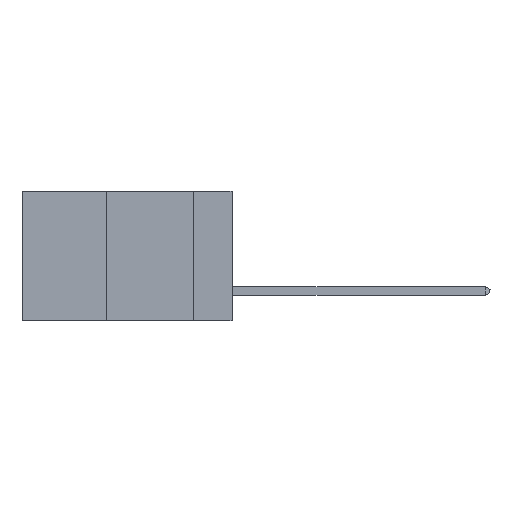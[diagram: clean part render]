
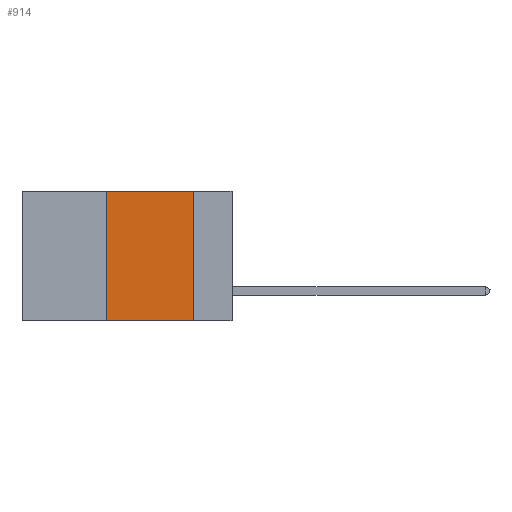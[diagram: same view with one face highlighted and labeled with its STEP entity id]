
A CAD part, left-side view. The second image highlights one B-rep face of the part: STEP entity #914.
In plain terms, the highlighted planar face has unit normal (-1, 0, 0).
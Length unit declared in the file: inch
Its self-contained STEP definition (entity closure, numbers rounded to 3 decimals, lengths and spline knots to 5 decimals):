
#914 = ADVANCED_FACE ( 'NONE', ( #29356 ), #25094, .F. ) ;
#1149 = DIRECTION ( 'NONE',  ( 0., 0., -1. ) ) ;
#3199 = DIRECTION ( 'NONE',  ( 0., -1., 0. ) ) ;
#3224 = LINE ( 'NONE', #44170, #32266 ) ;
#6078 = EDGE_CURVE ( 'NONE', #29932, #25414, #29934, .T. ) ;
#13713 = VECTOR ( 'NONE', #3199, 39.37008 ) ;
#16697 = AXIS2_PLACEMENT_3D ( 'NONE', #36150, #47114, #25277 ) ;
#17004 = DIRECTION ( 'NONE',  ( 0., 0., 1. ) ) ;
#17355 = VECTOR ( 'NONE', #1149, 39.37008 ) ;
#18553 = ORIENTED_EDGE ( 'NONE', *, *, #6078, .F. ) ;
#19811 = CARTESIAN_POINT ( 'NONE',  ( 0., 0.11, 0. ) ) ;
#20296 = DIRECTION ( 'NONE',  ( 0., -1., 0. ) ) ;
#22205 = LINE ( 'NONE', #19811, #17355 ) ;
#22661 = CARTESIAN_POINT ( 'NONE',  ( 0., 0.6, 0. ) ) ;
#22888 = CARTESIAN_POINT ( 'NONE',  ( 0., 0.36, 0. ) ) ;
#23502 = CARTESIAN_POINT ( 'NONE',  ( 0., 0.36, -0.37 ) ) ;
#25094 = PLANE ( 'NONE',  #16697 ) ;
#25143 = EDGE_CURVE ( 'NONE', #29932, #46502, #3224, .T. ) ;
#25277 = DIRECTION ( 'NONE',  ( 0., 0., -1. ) ) ;
#25414 = VERTEX_POINT ( 'NONE', #22888 ) ;
#25707 = ORIENTED_EDGE ( 'NONE', *, *, #34736, .F. ) ;
#25846 = EDGE_CURVE ( 'NONE', #36117, #46502, #22205, .T. ) ;
#29356 = FACE_OUTER_BOUND ( 'NONE', #30648, .T. ) ;
#29932 = VERTEX_POINT ( 'NONE', #23502 ) ;
#29934 = LINE ( 'NONE', #46549, #43376 ) ;
#30648 = EDGE_LOOP ( 'NONE', ( #37090, #25707, #18553, #37803 ) ) ;
#32266 = VECTOR ( 'NONE', #20296, 39.37008 ) ;
#34736 = EDGE_CURVE ( 'NONE', #25414, #36117, #47396, .T. ) ;
#36117 = VERTEX_POINT ( 'NONE', #48420 ) ;
#36150 = CARTESIAN_POINT ( 'NONE',  ( 0., 0.6, 0. ) ) ;
#37090 = ORIENTED_EDGE ( 'NONE', *, *, #25846, .F. ) ;
#37803 = ORIENTED_EDGE ( 'NONE', *, *, #25143, .T. ) ;
#38671 = CARTESIAN_POINT ( 'NONE',  ( 0., 0.11, -0.37 ) ) ;
#43376 = VECTOR ( 'NONE', #17004, 39.37008 ) ;
#44170 = CARTESIAN_POINT ( 'NONE',  ( 0., 0.6, -0.37 ) ) ;
#46502 = VERTEX_POINT ( 'NONE', #38671 ) ;
#46549 = CARTESIAN_POINT ( 'NONE',  ( 0., 0.36, 0. ) ) ;
#47114 = DIRECTION ( 'NONE',  ( 1., 0., 0. ) ) ;
#47396 = LINE ( 'NONE', #22661, #13713 ) ;
#48420 = CARTESIAN_POINT ( 'NONE',  ( 0., 0.11, 0. ) ) ;
